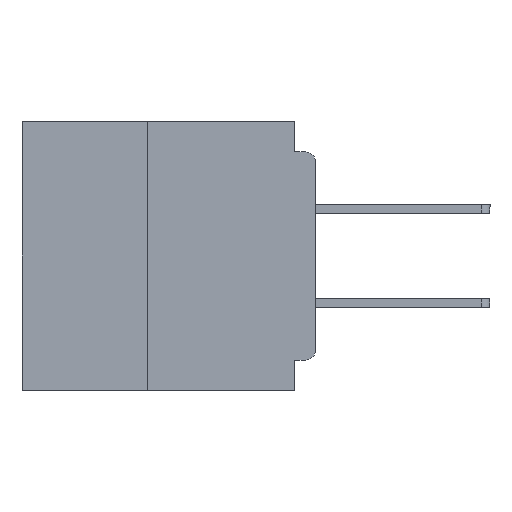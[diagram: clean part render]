
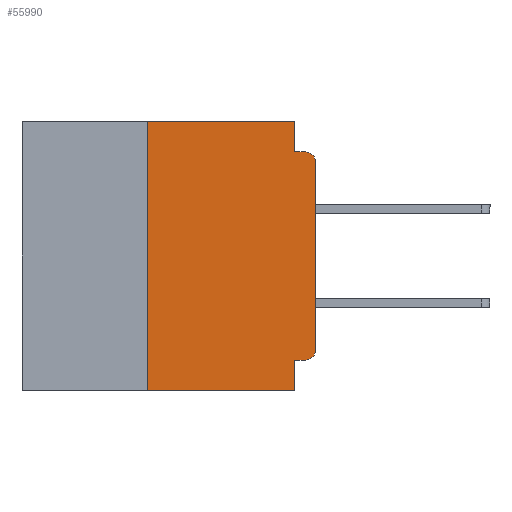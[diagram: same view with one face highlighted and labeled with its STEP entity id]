
A CAD part, left-side view. The second image highlights one B-rep face of the part: STEP entity #55990.
In plain terms, the highlighted planar face has unit normal (-1, 0, 0).
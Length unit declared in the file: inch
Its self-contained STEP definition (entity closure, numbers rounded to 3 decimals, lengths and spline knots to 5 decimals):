
#788 = DIRECTION ( 'NONE',  ( 0., 0., -1. ) ) ;
#1222 = VECTOR ( 'NONE', #23752, 39.37008 ) ;
#1415 = EDGE_CURVE ( 'NONE', #25346, #25063, #3519, .T. ) ;
#1595 = ORIENTED_EDGE ( 'NONE', *, *, #35202, .F. ) ;
#2908 = VERTEX_POINT ( 'NONE', #45360 ) ;
#3345 = EDGE_CURVE ( 'NONE', #2908, #48743, #36548, .T. ) ;
#3374 = CARTESIAN_POINT ( 'NONE',  ( 0., 0.437, 0. ) ) ;
#3519 = LINE ( 'NONE', #20852, #25691 ) ;
#4258 = ORIENTED_EDGE ( 'NONE', *, *, #3345, .F. ) ;
#4452 = VECTOR ( 'NONE', #49099, 39.37008 ) ;
#5092 = CARTESIAN_POINT ( 'NONE',  ( 0., 0.031, -0.355 ) ) ;
#5961 = CARTESIAN_POINT ( 'NONE',  ( 0., 0.015, -0.045 ) ) ;
#6749 = DIRECTION ( 'NONE',  ( 1., 0., 0. ) ) ;
#7427 = DIRECTION ( 'NONE',  ( 0., -1., 0. ) ) ;
#7462 = CARTESIAN_POINT ( 'NONE',  ( 0., 0.031, 0. ) ) ;
#7616 = FACE_OUTER_BOUND ( 'NONE', #12185, .T. ) ;
#8048 = CARTESIAN_POINT ( 'NONE',  ( 0., 0.015, -0.34 ) ) ;
#8272 = CARTESIAN_POINT ( 'NONE',  ( 0., 0., -0.045 ) ) ;
#8810 = LINE ( 'NONE', #3374, #38634 ) ;
#9659 = CARTESIAN_POINT ( 'NONE',  ( 0., 0.031, -0.4 ) ) ;
#10824 = CARTESIAN_POINT ( 'NONE',  ( 0., 0.25, 0. ) ) ;
#10877 = VECTOR ( 'NONE', #7427, 39.37008 ) ;
#11946 = DIRECTION ( 'NONE',  ( 0., 0., -1. ) ) ;
#12185 = EDGE_LOOP ( 'NONE', ( #42188, #16367, #44434, #1595, #16004, #4258, #32755, #29892, #52699, #27846 ) ) ;
#12531 = DIRECTION ( 'NONE',  ( 0., 0., -1. ) ) ;
#13812 = VERTEX_POINT ( 'NONE', #19080 ) ;
#13881 = CARTESIAN_POINT ( 'NONE',  ( 0., 0., -0.34 ) ) ;
#14389 = CARTESIAN_POINT ( 'NONE',  ( 0., 0., 0. ) ) ;
#15726 = VECTOR ( 'NONE', #27782, 39.37008 ) ;
#16004 = ORIENTED_EDGE ( 'NONE', *, *, #42436, .F. ) ;
#16367 = ORIENTED_EDGE ( 'NONE', *, *, #51349, .T. ) ;
#17339 = CARTESIAN_POINT ( 'NONE',  ( 0., 0., -0.06 ) ) ;
#17609 = AXIS2_PLACEMENT_3D ( 'NONE', #53764, #27303, #788 ) ;
#17861 = VECTOR ( 'NONE', #30568, 39.37008 ) ;
#18112 = CARTESIAN_POINT ( 'NONE',  ( 0., 0.031, -0.4 ) ) ;
#19080 = CARTESIAN_POINT ( 'NONE',  ( 0., 0.031, 0. ) ) ;
#19145 = VECTOR ( 'NONE', #11946, 39.37008 ) ;
#20603 = DIRECTION ( 'NONE',  ( 0., 1., 0. ) ) ;
#20852 = CARTESIAN_POINT ( 'NONE',  ( 0., 0., -0.355 ) ) ;
#22756 = EDGE_CURVE ( 'NONE', #48660, #28350, #42852, .T. ) ;
#23241 = CARTESIAN_POINT ( 'NONE',  ( 0., 0.031, -0.045 ) ) ;
#23752 = DIRECTION ( 'NONE',  ( 0., 0., 1. ) ) ;
#24980 = CARTESIAN_POINT ( 'NONE',  ( 0., 0.25, -0.4 ) ) ;
#25063 = VERTEX_POINT ( 'NONE', #5092 ) ;
#25346 = VERTEX_POINT ( 'NONE', #33528 ) ;
#25691 = VECTOR ( 'NONE', #20603, 39.37008 ) ;
#27207 = EDGE_CURVE ( 'NONE', #2908, #28251, #34481, .T. ) ;
#27303 = DIRECTION ( 'NONE',  ( -1., 0., 0. ) ) ;
#27574 = LINE ( 'NONE', #14389, #15726 ) ;
#27782 = DIRECTION ( 'NONE',  ( 0., 0., 1. ) ) ;
#27846 = ORIENTED_EDGE ( 'NONE', *, *, #33392, .T. ) ;
#28251 = VERTEX_POINT ( 'NONE', #9659 ) ;
#28350 = VERTEX_POINT ( 'NONE', #5961 ) ;
#28748 = VERTEX_POINT ( 'NONE', #17339 ) ;
#28831 = EDGE_CURVE ( 'NONE', #25063, #28251, #38436, .T. ) ;
#29892 = ORIENTED_EDGE ( 'NONE', *, *, #28831, .F. ) ;
#30459 = AXIS2_PLACEMENT_3D ( 'NONE', #33313, #6749, #37767 ) ;
#30568 = DIRECTION ( 'NONE',  ( 0., -1., 0. ) ) ;
#32755 = ORIENTED_EDGE ( 'NONE', *, *, #27207, .T. ) ;
#33313 = CARTESIAN_POINT ( 'NONE',  ( 0., 0.437, 0. ) ) ;
#33392 = EDGE_CURVE ( 'NONE', #25346, #57020, #53911, .T. ) ;
#33528 = CARTESIAN_POINT ( 'NONE',  ( 0., 0.015, -0.355 ) ) ;
#33803 = CARTESIAN_POINT ( 'NONE',  ( 0., 0.437, -0.4 ) ) ;
#34481 = LINE ( 'NONE', #33803, #10877 ) ;
#35202 = EDGE_CURVE ( 'NONE', #13812, #48660, #51703, .T. ) ;
#36548 = LINE ( 'NONE', #24980, #1222 ) ;
#37767 = DIRECTION ( 'NONE',  ( 0., 0., -1. ) ) ;
#38436 = LINE ( 'NONE', #18112, #4452 ) ;
#38634 = VECTOR ( 'NONE', #47924, 39.37008 ) ;
#39073 = DIRECTION ( 'NONE',  ( -1., 0., 0. ) ) ;
#42037 = CIRCLE ( 'NONE', #17609, 0.015 ) ;
#42188 = ORIENTED_EDGE ( 'NONE', *, *, #48007, .T. ) ;
#42436 = EDGE_CURVE ( 'NONE', #48743, #13812, #8810, .T. ) ;
#42852 = LINE ( 'NONE', #8272, #17861 ) ;
#44434 = ORIENTED_EDGE ( 'NONE', *, *, #22756, .F. ) ;
#45360 = CARTESIAN_POINT ( 'NONE',  ( 0., 0.25, -0.4 ) ) ;
#47924 = DIRECTION ( 'NONE',  ( 0., -1., 0. ) ) ;
#48007 = EDGE_CURVE ( 'NONE', #57020, #28748, #27574, .T. ) ;
#48660 = VERTEX_POINT ( 'NONE', #23241 ) ;
#48743 = VERTEX_POINT ( 'NONE', #10824 ) ;
#49099 = DIRECTION ( 'NONE',  ( 0., 0., -1. ) ) ;
#51349 = EDGE_CURVE ( 'NONE', #28748, #28350, #42037, .T. ) ;
#51703 = LINE ( 'NONE', #7462, #19145 ) ;
#52121 = AXIS2_PLACEMENT_3D ( 'NONE', #8048, #39073, #12531 ) ;
#52699 = ORIENTED_EDGE ( 'NONE', *, *, #1415, .F. ) ;
#53764 = CARTESIAN_POINT ( 'NONE',  ( 0., 0.015, -0.06 ) ) ;
#53911 = CIRCLE ( 'NONE', #52121, 0.015 ) ;
#55322 = PLANE ( 'NONE',  #30459 ) ;
#55990 = ADVANCED_FACE ( 'NONE', ( #7616 ), #55322, .F. ) ;
#57020 = VERTEX_POINT ( 'NONE', #13881 ) ;
